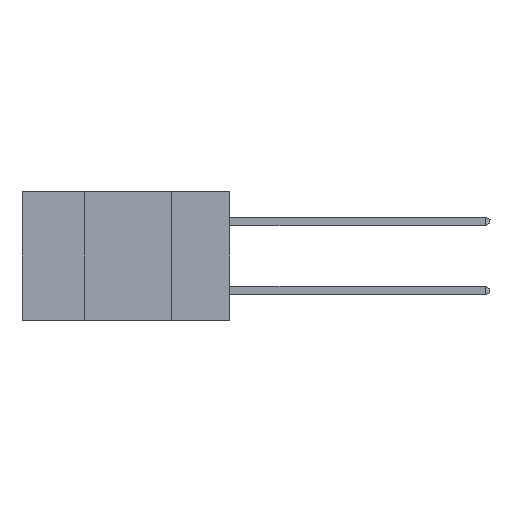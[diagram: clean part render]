
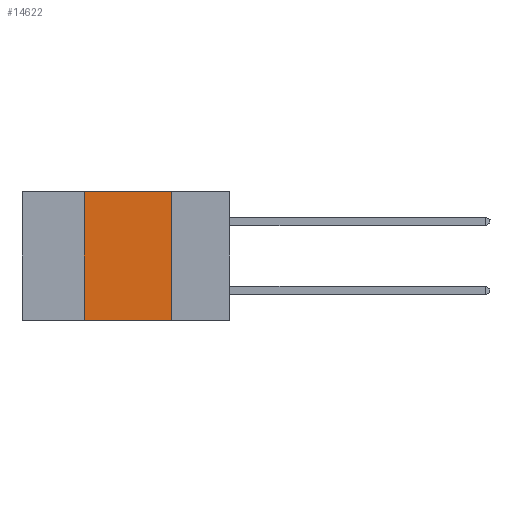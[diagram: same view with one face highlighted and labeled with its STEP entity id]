
A CAD part, left-side view. The second image highlights one B-rep face of the part: STEP entity #14622.
In plain terms, the highlighted planar face has unit normal (-1, 0, 0).
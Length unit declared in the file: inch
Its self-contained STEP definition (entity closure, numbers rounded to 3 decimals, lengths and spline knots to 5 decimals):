
#87 = ORIENTED_EDGE ( 'NONE', *, *, #11563, .F. ) ;
#279 = EDGE_CURVE ( 'NONE', #15271, #3780, #2285, .T. ) ;
#448 = AXIS2_PLACEMENT_3D ( 'NONE', #5304, #8625, #12279 ) ;
#1086 = LINE ( 'NONE', #7917, #15354 ) ;
#1884 = CARTESIAN_POINT ( 'NONE',  ( 0., 0.17, -0.37 ) ) ;
#2285 = LINE ( 'NONE', #12550, #9165 ) ;
#3385 = CARTESIAN_POINT ( 'NONE',  ( 0., 0.17, 0. ) ) ;
#3780 = VERTEX_POINT ( 'NONE', #3385 ) ;
#5196 = CARTESIAN_POINT ( 'NONE',  ( 0., 0.42, -0.37 ) ) ;
#5270 = CARTESIAN_POINT ( 'NONE',  ( 0., 0.42, 0. ) ) ;
#5304 = CARTESIAN_POINT ( 'NONE',  ( 0., 0.6, 0. ) ) ;
#5753 = DIRECTION ( 'NONE',  ( 0., -1., 0. ) ) ;
#7235 = PLANE ( 'NONE',  #448 ) ;
#7801 = DIRECTION ( 'NONE',  ( 0., 0., 1. ) ) ;
#7917 = CARTESIAN_POINT ( 'NONE',  ( 0., 0.42, -0.37 ) ) ;
#8194 = CARTESIAN_POINT ( 'NONE',  ( 0., 0.17, -0.37 ) ) ;
#8547 = VERTEX_POINT ( 'NONE', #5196 ) ;
#8625 = DIRECTION ( 'NONE',  ( 1., 0., 0. ) ) ;
#8744 = EDGE_CURVE ( 'NONE', #8547, #10388, #9523, .T. ) ;
#9165 = VECTOR ( 'NONE', #21673, 39.37008 ) ;
#9523 = LINE ( 'NONE', #21395, #10081 ) ;
#9535 = ORIENTED_EDGE ( 'NONE', *, *, #279, .F. ) ;
#10081 = VECTOR ( 'NONE', #5753, 39.37008 ) ;
#10388 = VERTEX_POINT ( 'NONE', #1884 ) ;
#11563 = EDGE_CURVE ( 'NONE', #8547, #15271, #1086, .T. ) ;
#12279 = DIRECTION ( 'NONE',  ( 0., 0., -1. ) ) ;
#12550 = CARTESIAN_POINT ( 'NONE',  ( 0., 0.6, 0. ) ) ;
#14622 = ADVANCED_FACE ( 'NONE', ( #21048 ), #7235, .F. ) ;
#14847 = EDGE_LOOP ( 'NONE', ( #20080, #9535, #87, #15330 ) ) ;
#15271 = VERTEX_POINT ( 'NONE', #5270 ) ;
#15330 = ORIENTED_EDGE ( 'NONE', *, *, #8744, .T. ) ;
#15354 = VECTOR ( 'NONE', #7801, 39.37008 ) ;
#17473 = EDGE_CURVE ( 'NONE', #3780, #10388, #18572, .T. ) ;
#17740 = VECTOR ( 'NONE', #18230, 39.37008 ) ;
#18230 = DIRECTION ( 'NONE',  ( 0., 0., -1. ) ) ;
#18572 = LINE ( 'NONE', #8194, #17740 ) ;
#20080 = ORIENTED_EDGE ( 'NONE', *, *, #17473, .F. ) ;
#21048 = FACE_OUTER_BOUND ( 'NONE', #14847, .T. ) ;
#21395 = CARTESIAN_POINT ( 'NONE',  ( 0., 0.6, -0.37 ) ) ;
#21673 = DIRECTION ( 'NONE',  ( 0., -1., 0. ) ) ;
